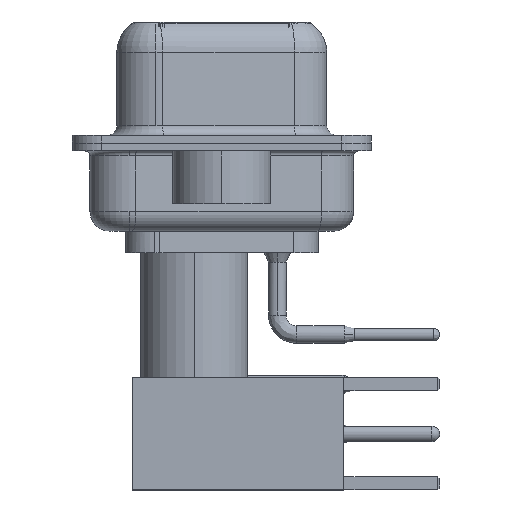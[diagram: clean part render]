
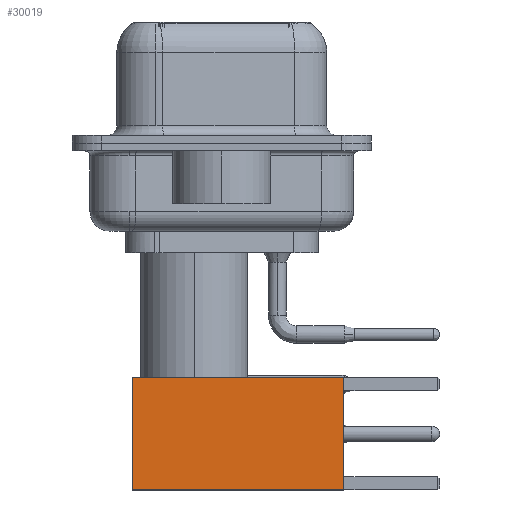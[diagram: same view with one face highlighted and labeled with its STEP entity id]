
A CAD part, left-side view. The second image highlights one B-rep face of the part: STEP entity #30019.
In plain terms, the highlighted face is planar.
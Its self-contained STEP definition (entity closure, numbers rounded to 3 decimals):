
#1916 = ORIENTED_EDGE ( 'NONE', *, *, #19184, .T. ) ;
#2151 = CARTESIAN_POINT ( 'NONE',  ( 0., 2.875, 10.82 ) ) ;
#6976 = PLANE ( 'NONE',  #9458 ) ;
#7024 = ORIENTED_EDGE ( 'NONE', *, *, #19731, .F. ) ;
#7167 = FACE_OUTER_BOUND ( 'NONE', #25389, .T. ) ;
#9458 = AXIS2_PLACEMENT_3D ( 'NONE', #21423, #23898, #18436 ) ;
#9740 = LINE ( 'NONE', #26268, #28729 ) ;
#11660 = LINE ( 'NONE', #17101, #18615 ) ;
#15608 = DIRECTION ( 'NONE',  ( -1., 0., 0. ) ) ;
#16066 = ORIENTED_EDGE ( 'NONE', *, *, #23077, .T. ) ;
#16083 = CARTESIAN_POINT ( 'NONE',  ( -2.875, 2.875, 10.82 ) ) ;
#17027 = CARTESIAN_POINT ( 'NONE',  ( 2.875, 2.875, 10.82 ) ) ;
#17101 = CARTESIAN_POINT ( 'NONE',  ( 2.875, 2.875, 0. ) ) ;
#17281 = VECTOR ( 'NONE', #30883, 1000. ) ;
#18436 = DIRECTION ( 'NONE',  ( 0., 0., 1. ) ) ;
#18615 = VECTOR ( 'NONE', #28952, 1000. ) ;
#19184 = EDGE_CURVE ( 'NONE', #31032, #24143, #20851, .T. ) ;
#19435 = LINE ( 'NONE', #2151, #17281 ) ;
#19731 = EDGE_CURVE ( 'NONE', #21286, #27840, #19435, .T. ) ;
#20851 = LINE ( 'NONE', #29861, #35230 ) ;
#20907 = ORIENTED_EDGE ( 'NONE', *, *, #22390, .F. ) ;
#21286 = VERTEX_POINT ( 'NONE', #17027 ) ;
#21423 = CARTESIAN_POINT ( 'NONE',  ( 2.875, 2.875, 0. ) ) ;
#22390 = EDGE_CURVE ( 'NONE', #27840, #24143, #9740, .T. ) ;
#23077 = EDGE_CURVE ( 'NONE', #21286, #31032, #11660, .T. ) ;
#23607 = CARTESIAN_POINT ( 'NONE',  ( -2.875, 2.875, 0. ) ) ;
#23898 = DIRECTION ( 'NONE',  ( 0., 1., 0. ) ) ;
#24143 = VERTEX_POINT ( 'NONE', #23607 ) ;
#25389 = EDGE_LOOP ( 'NONE', ( #16066, #1916, #20907, #7024 ) ) ;
#26268 = CARTESIAN_POINT ( 'NONE',  ( -2.875, 2.875, 0. ) ) ;
#26831 = DIRECTION ( 'NONE',  ( 0., 0., -1. ) ) ;
#27840 = VERTEX_POINT ( 'NONE', #16083 ) ;
#28729 = VECTOR ( 'NONE', #26831, 1000. ) ;
#28952 = DIRECTION ( 'NONE',  ( 0., 0., -1. ) ) ;
#29861 = CARTESIAN_POINT ( 'NONE',  ( 0., 2.875, 0. ) ) ;
#30019 = ADVANCED_FACE ( 'NONE', ( #7167 ), #6976, .T. ) ;
#30883 = DIRECTION ( 'NONE',  ( -1., 0., 0. ) ) ;
#31032 = VERTEX_POINT ( 'NONE', #37069 ) ;
#35230 = VECTOR ( 'NONE', #15608, 1000. ) ;
#37069 = CARTESIAN_POINT ( 'NONE',  ( 2.875, 2.875, 0. ) ) ;
